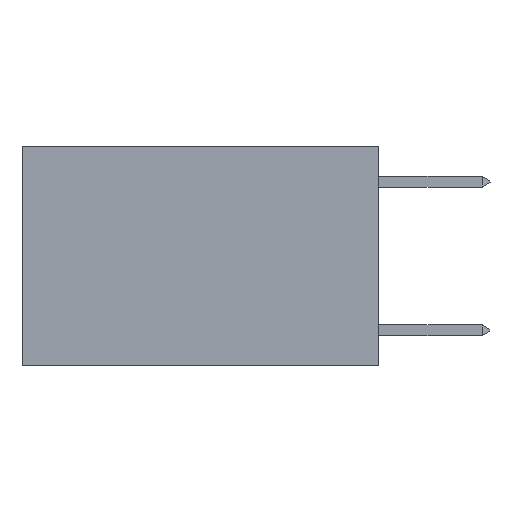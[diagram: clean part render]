
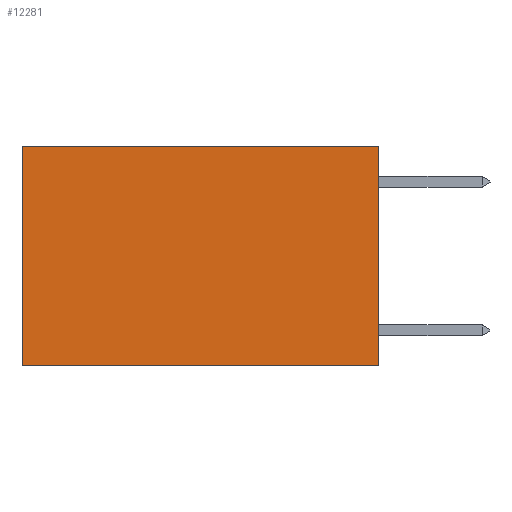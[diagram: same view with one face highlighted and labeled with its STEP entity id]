
A CAD part, left-side view. The second image highlights one B-rep face of the part: STEP entity #12281.
In plain terms, the highlighted planar face has unit normal (-1, 0, 0).
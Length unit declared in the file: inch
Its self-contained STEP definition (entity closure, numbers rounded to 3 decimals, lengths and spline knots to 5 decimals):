
#2150 = VECTOR ( 'NONE', #8790, 39.37008 ) ;
#3295 = AXIS2_PLACEMENT_3D ( 'NONE', #17193, #11179, #20921 ) ;
#3827 = DIRECTION ( 'NONE',  ( 0., 1., 0. ) ) ;
#5387 = VERTEX_POINT ( 'NONE', #15362 ) ;
#6117 = VECTOR ( 'NONE', #11433, 39.37008 ) ;
#7287 = PLANE ( 'NONE',  #3295 ) ;
#7352 = VERTEX_POINT ( 'NONE', #15004 ) ;
#7457 = CARTESIAN_POINT ( 'NONE',  ( 0.2625, 0., -0.37 ) ) ;
#8128 = LINE ( 'NONE', #15603, #12731 ) ;
#8790 = DIRECTION ( 'NONE',  ( 0., 0., -1. ) ) ;
#10718 = CARTESIAN_POINT ( 'NONE',  ( 0.2625, 0.6, 0. ) ) ;
#11179 = DIRECTION ( 'NONE',  ( 1., 0., 0. ) ) ;
#11224 = ORIENTED_EDGE ( 'NONE', *, *, #17883, .F. ) ;
#11433 = DIRECTION ( 'NONE',  ( 0., 1., 0. ) ) ;
#11521 = VERTEX_POINT ( 'NONE', #23803 ) ;
#12281 = ADVANCED_FACE ( 'NONE', ( #12907 ), #7287, .F. ) ;
#12731 = VECTOR ( 'NONE', #3827, 39.37008 ) ;
#12907 = FACE_OUTER_BOUND ( 'NONE', #16318, .T. ) ;
#12946 = EDGE_CURVE ( 'NONE', #5387, #15571, #15535, .T. ) ;
#13877 = DIRECTION ( 'NONE',  ( 0., 0., -1. ) ) ;
#14715 = LINE ( 'NONE', #16796, #2150 ) ;
#15004 = CARTESIAN_POINT ( 'NONE',  ( 0.2625, 0., -0.37 ) ) ;
#15362 = CARTESIAN_POINT ( 'NONE',  ( 0.2625, 0.6, 0. ) ) ;
#15535 = LINE ( 'NONE', #10718, #15820 ) ;
#15571 = VERTEX_POINT ( 'NONE', #18013 ) ;
#15603 = CARTESIAN_POINT ( 'NONE',  ( 0.2625, 0., 0. ) ) ;
#15820 = VECTOR ( 'NONE', #13877, 39.37008 ) ;
#16318 = EDGE_LOOP ( 'NONE', ( #18554, #11224, #24313, #18648 ) ) ;
#16796 = CARTESIAN_POINT ( 'NONE',  ( 0.2625, 0., 0. ) ) ;
#17193 = CARTESIAN_POINT ( 'NONE',  ( 0.2625, 0., 0. ) ) ;
#17515 = EDGE_CURVE ( 'NONE', #11521, #7352, #14715, .T. ) ;
#17883 = EDGE_CURVE ( 'NONE', #7352, #15571, #19881, .T. ) ;
#18013 = CARTESIAN_POINT ( 'NONE',  ( 0.2625, 0.6, -0.37 ) ) ;
#18554 = ORIENTED_EDGE ( 'NONE', *, *, #12946, .T. ) ;
#18648 = ORIENTED_EDGE ( 'NONE', *, *, #24337, .T. ) ;
#19881 = LINE ( 'NONE', #7457, #6117 ) ;
#20921 = DIRECTION ( 'NONE',  ( 0., 0., -1. ) ) ;
#23803 = CARTESIAN_POINT ( 'NONE',  ( 0.2625, 0., 0. ) ) ;
#24313 = ORIENTED_EDGE ( 'NONE', *, *, #17515, .F. ) ;
#24337 = EDGE_CURVE ( 'NONE', #11521, #5387, #8128, .T. ) ;
